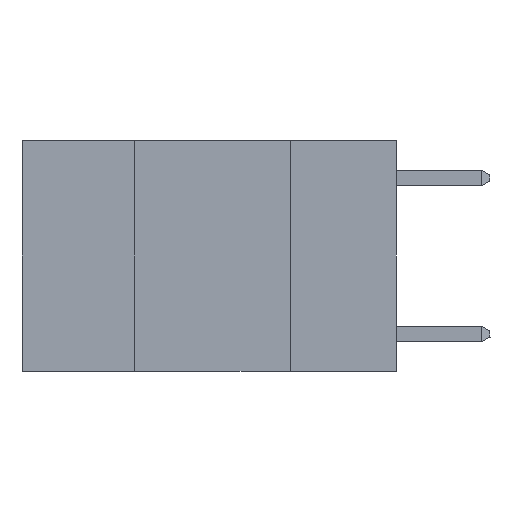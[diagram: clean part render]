
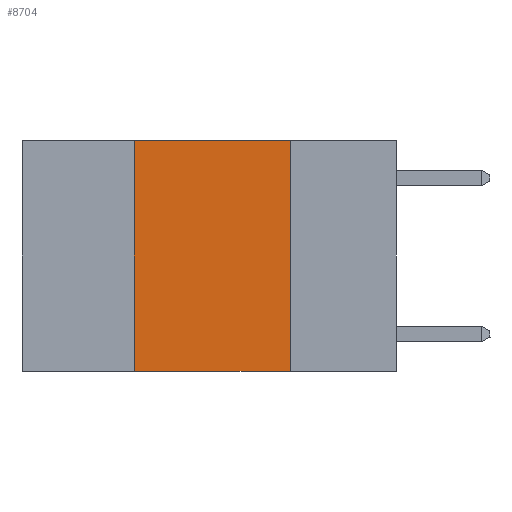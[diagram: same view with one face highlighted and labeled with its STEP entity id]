
A CAD part, left-side view. The second image highlights one B-rep face of the part: STEP entity #8704.
In plain terms, the highlighted planar face has unit normal (-1, 0, 0).
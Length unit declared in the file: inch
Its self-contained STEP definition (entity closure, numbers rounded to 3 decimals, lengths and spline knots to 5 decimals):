
#260 = EDGE_CURVE ( 'NONE', #7776, #3473, #3301, .T. ) ;
#543 = VECTOR ( 'NONE', #1167, 39.37008 ) ;
#1167 = DIRECTION ( 'NONE',  ( 0., 0., 1. ) ) ;
#2895 = CARTESIAN_POINT ( 'NONE',  ( 0., 0.42, 0. ) ) ;
#2964 = CARTESIAN_POINT ( 'NONE',  ( 0., 0.6, 0. ) ) ;
#3034 = EDGE_LOOP ( 'NONE', ( #8753, #5680, #10632, #8188 ) ) ;
#3078 = LINE ( 'NONE', #4460, #543 ) ;
#3266 = EDGE_CURVE ( 'NONE', #7039, #3473, #8054, .T. ) ;
#3301 = LINE ( 'NONE', #7351, #5229 ) ;
#3330 = FACE_OUTER_BOUND ( 'NONE', #3034, .T. ) ;
#3411 = CARTESIAN_POINT ( 'NONE',  ( 0., 0.6, 0. ) ) ;
#3473 = VERTEX_POINT ( 'NONE', #4055 ) ;
#3940 = CARTESIAN_POINT ( 'NONE',  ( 0., 0.42, -0.37 ) ) ;
#3941 = EDGE_CURVE ( 'NONE', #9523, #7039, #6287, .T. ) ;
#4055 = CARTESIAN_POINT ( 'NONE',  ( 0., 0.17, -0.37 ) ) ;
#4093 = VECTOR ( 'NONE', #10228, 39.37008 ) ;
#4207 = DIRECTION ( 'NONE',  ( 1., 0., 0. ) ) ;
#4303 = DIRECTION ( 'NONE',  ( 0., -1., 0. ) ) ;
#4460 = CARTESIAN_POINT ( 'NONE',  ( 0., 0.42, 0. ) ) ;
#5229 = VECTOR ( 'NONE', #4303, 39.37008 ) ;
#5680 = ORIENTED_EDGE ( 'NONE', *, *, #3941, .F. ) ;
#5919 = VECTOR ( 'NONE', #8673, 39.37008 ) ;
#6287 = LINE ( 'NONE', #2964, #4093 ) ;
#7039 = VERTEX_POINT ( 'NONE', #9580 ) ;
#7331 = AXIS2_PLACEMENT_3D ( 'NONE', #3411, #4207, #9842 ) ;
#7351 = CARTESIAN_POINT ( 'NONE',  ( 0., 0.6, -0.37 ) ) ;
#7776 = VERTEX_POINT ( 'NONE', #3940 ) ;
#7872 = CARTESIAN_POINT ( 'NONE',  ( 0., 0.17, 0. ) ) ;
#8054 = LINE ( 'NONE', #7872, #5919 ) ;
#8188 = ORIENTED_EDGE ( 'NONE', *, *, #260, .T. ) ;
#8252 = PLANE ( 'NONE',  #7331 ) ;
#8673 = DIRECTION ( 'NONE',  ( 0., 0., -1. ) ) ;
#8704 = ADVANCED_FACE ( 'NONE', ( #3330 ), #8252, .F. ) ;
#8753 = ORIENTED_EDGE ( 'NONE', *, *, #3266, .F. ) ;
#8878 = EDGE_CURVE ( 'NONE', #7776, #9523, #3078, .T. ) ;
#9523 = VERTEX_POINT ( 'NONE', #2895 ) ;
#9580 = CARTESIAN_POINT ( 'NONE',  ( 0., 0.17, 0. ) ) ;
#9842 = DIRECTION ( 'NONE',  ( 0., 0., -1. ) ) ;
#10228 = DIRECTION ( 'NONE',  ( 0., -1., 0. ) ) ;
#10632 = ORIENTED_EDGE ( 'NONE', *, *, #8878, .F. ) ;
